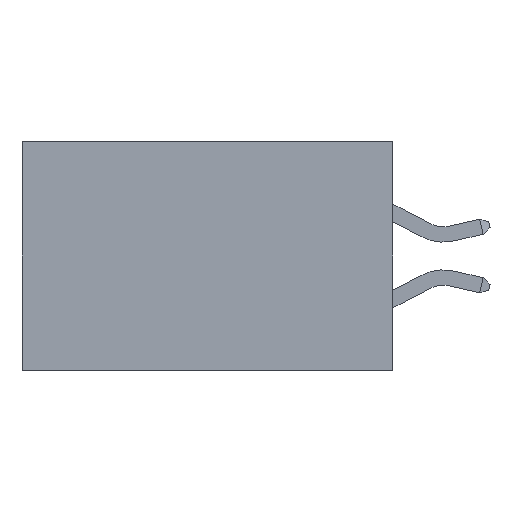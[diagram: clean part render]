
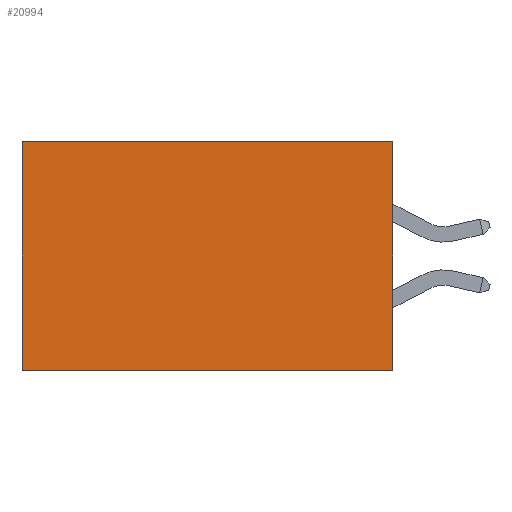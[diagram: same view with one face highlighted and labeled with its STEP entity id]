
A CAD part, left-side view. The second image highlights one B-rep face of the part: STEP entity #20994.
In plain terms, the highlighted planar face has unit normal (-1, 0, 0).
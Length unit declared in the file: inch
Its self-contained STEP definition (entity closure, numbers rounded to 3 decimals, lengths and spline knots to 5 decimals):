
#1957 = EDGE_CURVE ( 'NONE', #31661, #11426, #31765, .T. ) ;
#3567 = LINE ( 'NONE', #20600, #5818 ) ;
#5178 = CARTESIAN_POINT ( 'NONE',  ( 0.2875, 0., 0. ) ) ;
#5818 = VECTOR ( 'NONE', #14789, 39.37008 ) ;
#6450 = ORIENTED_EDGE ( 'NONE', *, *, #19890, .T. ) ;
#7435 = DIRECTION ( 'NONE',  ( 0., 0., -1. ) ) ;
#8652 = VECTOR ( 'NONE', #7435, 39.37008 ) ;
#8861 = DIRECTION ( 'NONE',  ( 0., 0., -1. ) ) ;
#8981 = CARTESIAN_POINT ( 'NONE',  ( 0.2875, 0., 0. ) ) ;
#9103 = PLANE ( 'NONE',  #13817 ) ;
#9785 = EDGE_CURVE ( 'NONE', #31661, #21543, #35335, .T. ) ;
#10000 = CARTESIAN_POINT ( 'NONE',  ( 0.2875, 0., -0.37 ) ) ;
#11426 = VERTEX_POINT ( 'NONE', #10000 ) ;
#13817 = AXIS2_PLACEMENT_3D ( 'NONE', #8981, #17712, #8861 ) ;
#14789 = DIRECTION ( 'NONE',  ( 0., 1., 0. ) ) ;
#15214 = LINE ( 'NONE', #27414, #29739 ) ;
#17712 = DIRECTION ( 'NONE',  ( 1., 0., 0. ) ) ;
#18366 = VERTEX_POINT ( 'NONE', #31481 ) ;
#18924 = CARTESIAN_POINT ( 'NONE',  ( 0.2875, 0.6, 0. ) ) ;
#19232 = FACE_OUTER_BOUND ( 'NONE', #22053, .T. ) ;
#19890 = EDGE_CURVE ( 'NONE', #21543, #18366, #15214, .T. ) ;
#20600 = CARTESIAN_POINT ( 'NONE',  ( 0.2875, 0., -0.37 ) ) ;
#20994 = ADVANCED_FACE ( 'NONE', ( #19232 ), #9103, .F. ) ;
#21543 = VERTEX_POINT ( 'NONE', #18924 ) ;
#22053 = EDGE_LOOP ( 'NONE', ( #6450, #30010, #37130, #30444 ) ) ;
#24463 = VECTOR ( 'NONE', #27960, 39.37008 ) ;
#27414 = CARTESIAN_POINT ( 'NONE',  ( 0.2875, 0.6, 0. ) ) ;
#27417 = CARTESIAN_POINT ( 'NONE',  ( 0.2875, 0., 0. ) ) ;
#27453 = CARTESIAN_POINT ( 'NONE',  ( 0.2875, 0., 0. ) ) ;
#27960 = DIRECTION ( 'NONE',  ( 0., 1., 0. ) ) ;
#29739 = VECTOR ( 'NONE', #30070, 39.37008 ) ;
#30010 = ORIENTED_EDGE ( 'NONE', *, *, #30571, .F. ) ;
#30070 = DIRECTION ( 'NONE',  ( 0., 0., -1. ) ) ;
#30444 = ORIENTED_EDGE ( 'NONE', *, *, #9785, .T. ) ;
#30571 = EDGE_CURVE ( 'NONE', #11426, #18366, #3567, .T. ) ;
#31481 = CARTESIAN_POINT ( 'NONE',  ( 0.2875, 0.6, -0.37 ) ) ;
#31661 = VERTEX_POINT ( 'NONE', #27453 ) ;
#31765 = LINE ( 'NONE', #27417, #8652 ) ;
#35335 = LINE ( 'NONE', #5178, #24463 ) ;
#37130 = ORIENTED_EDGE ( 'NONE', *, *, #1957, .F. ) ;
